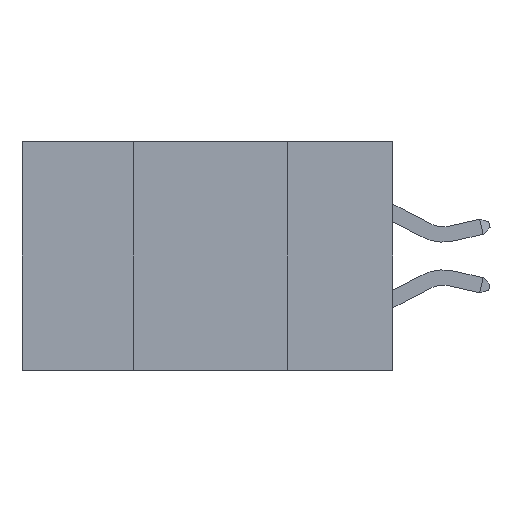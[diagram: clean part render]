
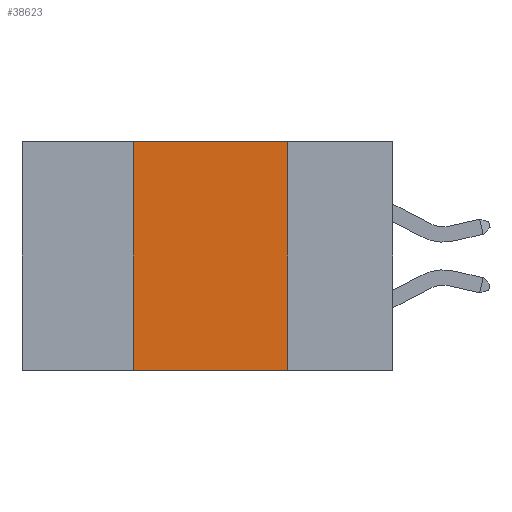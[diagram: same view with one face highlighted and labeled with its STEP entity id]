
A CAD part, left-side view. The second image highlights one B-rep face of the part: STEP entity #38623.
In plain terms, the highlighted planar face has unit normal (-1, 0, 0).
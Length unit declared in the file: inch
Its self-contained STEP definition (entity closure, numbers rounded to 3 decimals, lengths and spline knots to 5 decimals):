
#781 = VECTOR ( 'NONE', #14041, 39.37008 ) ;
#2141 = VECTOR ( 'NONE', #32510, 39.37008 ) ;
#5537 = LINE ( 'NONE', #39046, #21059 ) ;
#5745 = DIRECTION ( 'NONE',  ( 0., -1., 0. ) ) ;
#9062 = CARTESIAN_POINT ( 'NONE',  ( 0., 0.17, -0.37 ) ) ;
#9429 = VERTEX_POINT ( 'NONE', #40813 ) ;
#9614 = LINE ( 'NONE', #33843, #781 ) ;
#9867 = DIRECTION ( 'NONE',  ( 0., 0., -1. ) ) ;
#10907 = CARTESIAN_POINT ( 'NONE',  ( 0., 0.17, 0. ) ) ;
#11978 = ORIENTED_EDGE ( 'NONE', *, *, #24251, .F. ) ;
#14041 = DIRECTION ( 'NONE',  ( 0., 0., -1. ) ) ;
#14596 = EDGE_CURVE ( 'NONE', #9429, #23381, #36360, .T. ) ;
#16396 = CARTESIAN_POINT ( 'NONE',  ( 0., 0.6, 0. ) ) ;
#16514 = VERTEX_POINT ( 'NONE', #9062 ) ;
#20139 = ORIENTED_EDGE ( 'NONE', *, *, #23197, .T. ) ;
#20757 = CARTESIAN_POINT ( 'NONE',  ( 0., 0.42, -0.37 ) ) ;
#21059 = VECTOR ( 'NONE', #5745, 39.37008 ) ;
#23197 = EDGE_CURVE ( 'NONE', #23393, #16514, #5537, .T. ) ;
#23381 = VERTEX_POINT ( 'NONE', #10907 ) ;
#23393 = VERTEX_POINT ( 'NONE', #20757 ) ;
#24251 = EDGE_CURVE ( 'NONE', #23381, #16514, #9614, .T. ) ;
#24523 = CARTESIAN_POINT ( 'NONE',  ( 0., 0.42, 0. ) ) ;
#25791 = AXIS2_PLACEMENT_3D ( 'NONE', #36252, #42931, #9867 ) ;
#25808 = LINE ( 'NONE', #24523, #36667 ) ;
#26541 = EDGE_LOOP ( 'NONE', ( #11978, #35739, #27500, #20139 ) ) ;
#27500 = ORIENTED_EDGE ( 'NONE', *, *, #28401, .F. ) ;
#27826 = DIRECTION ( 'NONE',  ( 0., 0., 1. ) ) ;
#28401 = EDGE_CURVE ( 'NONE', #23393, #9429, #25808, .T. ) ;
#30859 = FACE_OUTER_BOUND ( 'NONE', #26541, .T. ) ;
#32510 = DIRECTION ( 'NONE',  ( 0., -1., 0. ) ) ;
#33843 = CARTESIAN_POINT ( 'NONE',  ( 0., 0.17, 0. ) ) ;
#35739 = ORIENTED_EDGE ( 'NONE', *, *, #14596, .F. ) ;
#36252 = CARTESIAN_POINT ( 'NONE',  ( 0., 0.6, 0. ) ) ;
#36360 = LINE ( 'NONE', #16396, #2141 ) ;
#36667 = VECTOR ( 'NONE', #27826, 39.37008 ) ;
#38623 = ADVANCED_FACE ( 'NONE', ( #30859 ), #39712, .F. ) ;
#39046 = CARTESIAN_POINT ( 'NONE',  ( 0., 0.6, -0.37 ) ) ;
#39712 = PLANE ( 'NONE',  #25791 ) ;
#40813 = CARTESIAN_POINT ( 'NONE',  ( 0., 0.42, 0. ) ) ;
#42931 = DIRECTION ( 'NONE',  ( 1., 0., 0. ) ) ;
